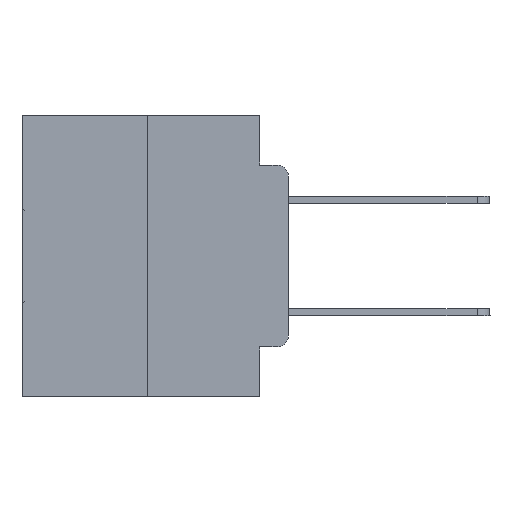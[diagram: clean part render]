
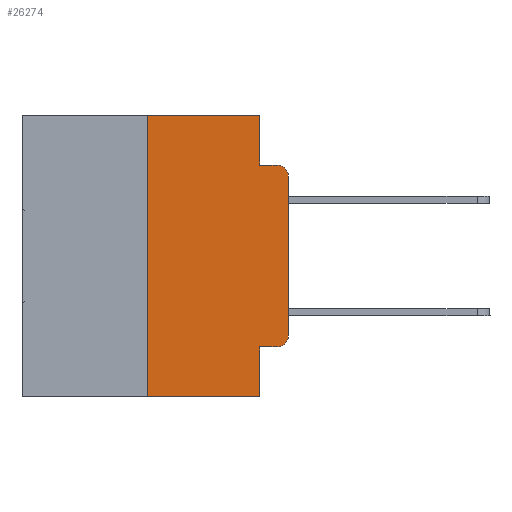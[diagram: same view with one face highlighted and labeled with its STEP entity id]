
A CAD part, left-side view. The second image highlights one B-rep face of the part: STEP entity #26274.
In plain terms, the highlighted planar face has unit normal (-1, 0, 0).
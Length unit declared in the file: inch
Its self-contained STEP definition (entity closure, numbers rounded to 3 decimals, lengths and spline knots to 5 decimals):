
#2 = CARTESIAN_POINT ( 'NONE',  ( 0., 0.051, -0.4115 ) ) ;
#1365 = CARTESIAN_POINT ( 'NONE',  ( 0., 0.051, 0. ) ) ;
#1436 = DIRECTION ( 'NONE',  ( -1., 0., 0. ) ) ;
#1447 = VECTOR ( 'NONE', #6251, 39.37008 ) ;
#1480 = DIRECTION ( 'NONE',  ( 0., 0., -1. ) ) ;
#2574 = DIRECTION ( 'NONE',  ( 0., -1., 0. ) ) ;
#2601 = LINE ( 'NONE', #25767, #10209 ) ;
#2672 = VECTOR ( 'NONE', #25219, 39.37008 ) ;
#3342 = CARTESIAN_POINT ( 'NONE',  ( 0., 0.473, -0.5 ) ) ;
#3492 = VERTEX_POINT ( 'NONE', #8586 ) ;
#4495 = ORIENTED_EDGE ( 'NONE', *, *, #32081, .T. ) ;
#4887 = LINE ( 'NONE', #1365, #26101 ) ;
#4944 = VECTOR ( 'NONE', #2574, 39.37008 ) ;
#5983 = EDGE_CURVE ( 'NONE', #24963, #23833, #2601, .T. ) ;
#6019 = CARTESIAN_POINT ( 'NONE',  ( 0., 0.051, -0.0885 ) ) ;
#6251 = DIRECTION ( 'NONE',  ( 0., -1., 0. ) ) ;
#7625 = CARTESIAN_POINT ( 'NONE',  ( 0., 0.051, -0.0885 ) ) ;
#8046 = VECTOR ( 'NONE', #30836, 39.37008 ) ;
#8366 = CARTESIAN_POINT ( 'NONE',  ( 0., 0.051, -0.4115 ) ) ;
#8586 = CARTESIAN_POINT ( 'NONE',  ( 0., 0., -0.3915 ) ) ;
#8615 = VERTEX_POINT ( 'NONE', #16525 ) ;
#8672 = CARTESIAN_POINT ( 'NONE',  ( 0., 0.473, 0. ) ) ;
#9557 = ORIENTED_EDGE ( 'NONE', *, *, #26837, .T. ) ;
#10017 = DIRECTION ( 'NONE',  ( -1., 0., 0. ) ) ;
#10176 = ORIENTED_EDGE ( 'NONE', *, *, #13258, .F. ) ;
#10209 = VECTOR ( 'NONE', #20400, 39.37008 ) ;
#10474 = AXIS2_PLACEMENT_3D ( 'NONE', #28047, #10017, #20224 ) ;
#12135 = AXIS2_PLACEMENT_3D ( 'NONE', #26826, #1436, #16648 ) ;
#12227 = VECTOR ( 'NONE', #26302, 39.37008 ) ;
#12442 = CARTESIAN_POINT ( 'NONE',  ( 0., 0.25, -0.5 ) ) ;
#12909 = CARTESIAN_POINT ( 'NONE',  ( 0., 0.02, -0.4115 ) ) ;
#13196 = EDGE_CURVE ( 'NONE', #17212, #8615, #16471, .T. ) ;
#13258 = EDGE_CURVE ( 'NONE', #15670, #23343, #27294, .T. ) ;
#14021 = ORIENTED_EDGE ( 'NONE', *, *, #20124, .T. ) ;
#15471 = LINE ( 'NONE', #8366, #1447 ) ;
#15670 = VERTEX_POINT ( 'NONE', #2 ) ;
#16412 = DIRECTION ( 'NONE',  ( 0., 0., -1. ) ) ;
#16471 = CIRCLE ( 'NONE', #10474, 0.02 ) ;
#16525 = CARTESIAN_POINT ( 'NONE',  ( 0., 0.02, -0.0885 ) ) ;
#16648 = DIRECTION ( 'NONE',  ( 0., 0., -1. ) ) ;
#17212 = VERTEX_POINT ( 'NONE', #27606 ) ;
#18235 = LINE ( 'NONE', #18359, #28618 ) ;
#18359 = CARTESIAN_POINT ( 'NONE',  ( 0., 0., 0. ) ) ;
#19729 = ORIENTED_EDGE ( 'NONE', *, *, #13196, .T. ) ;
#19916 = CARTESIAN_POINT ( 'NONE',  ( 0., 0.051, 0. ) ) ;
#20124 = EDGE_CURVE ( 'NONE', #28458, #23343, #22621, .T. ) ;
#20161 = VERTEX_POINT ( 'NONE', #6019 ) ;
#20224 = DIRECTION ( 'NONE',  ( 0., 0., -1. ) ) ;
#20400 = DIRECTION ( 'NONE',  ( 0., -1., 0. ) ) ;
#20582 = ORIENTED_EDGE ( 'NONE', *, *, #5983, .F. ) ;
#20632 = VERTEX_POINT ( 'NONE', #12909 ) ;
#21016 = ORIENTED_EDGE ( 'NONE', *, *, #22780, .F. ) ;
#21095 = EDGE_CURVE ( 'NONE', #20161, #8615, #23353, .T. ) ;
#22062 = ORIENTED_EDGE ( 'NONE', *, *, #23062, .T. ) ;
#22621 = LINE ( 'NONE', #3342, #12227 ) ;
#22780 = EDGE_CURVE ( 'NONE', #23833, #20161, #4887, .T. ) ;
#23062 = EDGE_CURVE ( 'NONE', #15670, #20632, #15471, .T. ) ;
#23343 = VERTEX_POINT ( 'NONE', #30082 ) ;
#23353 = LINE ( 'NONE', #7625, #4944 ) ;
#23796 = ORIENTED_EDGE ( 'NONE', *, *, #30231, .F. ) ;
#23833 = VERTEX_POINT ( 'NONE', #19916 ) ;
#23997 = PLANE ( 'NONE',  #29926 ) ;
#24219 = DIRECTION ( 'NONE',  ( 1., 0., 0. ) ) ;
#24963 = VERTEX_POINT ( 'NONE', #29328 ) ;
#25219 = DIRECTION ( 'NONE',  ( 0., 0., 1. ) ) ;
#25767 = CARTESIAN_POINT ( 'NONE',  ( 0., 0.473, 0. ) ) ;
#26074 = DIRECTION ( 'NONE',  ( 0., 0., 1. ) ) ;
#26101 = VECTOR ( 'NONE', #1480, 39.37008 ) ;
#26274 = ADVANCED_FACE ( 'NONE', ( #27096 ), #23997, .F. ) ;
#26302 = DIRECTION ( 'NONE',  ( 0., -1., 0. ) ) ;
#26826 = CARTESIAN_POINT ( 'NONE',  ( 0., 0.02, -0.3915 ) ) ;
#26837 = EDGE_CURVE ( 'NONE', #20632, #3492, #29080, .T. ) ;
#27096 = FACE_OUTER_BOUND ( 'NONE', #29685, .T. ) ;
#27294 = LINE ( 'NONE', #32991, #8046 ) ;
#27606 = CARTESIAN_POINT ( 'NONE',  ( 0., 0., -0.1085 ) ) ;
#28047 = CARTESIAN_POINT ( 'NONE',  ( 0., 0.02, -0.1085 ) ) ;
#28114 = ORIENTED_EDGE ( 'NONE', *, *, #21095, .F. ) ;
#28458 = VERTEX_POINT ( 'NONE', #12442 ) ;
#28618 = VECTOR ( 'NONE', #26074, 39.37008 ) ;
#29080 = CIRCLE ( 'NONE', #12135, 0.02 ) ;
#29328 = CARTESIAN_POINT ( 'NONE',  ( 0., 0.25, 0. ) ) ;
#29685 = EDGE_LOOP ( 'NONE', ( #4495, #19729, #28114, #21016, #20582, #23796, #14021, #10176, #22062, #9557 ) ) ;
#29926 = AXIS2_PLACEMENT_3D ( 'NONE', #8672, #24219, #16412 ) ;
#30082 = CARTESIAN_POINT ( 'NONE',  ( 0., 0.051, -0.5 ) ) ;
#30123 = CARTESIAN_POINT ( 'NONE',  ( 0., 0.25, 0. ) ) ;
#30231 = EDGE_CURVE ( 'NONE', #28458, #24963, #30728, .T. ) ;
#30728 = LINE ( 'NONE', #30123, #2672 ) ;
#30836 = DIRECTION ( 'NONE',  ( 0., 0., -1. ) ) ;
#32081 = EDGE_CURVE ( 'NONE', #3492, #17212, #18235, .T. ) ;
#32991 = CARTESIAN_POINT ( 'NONE',  ( 0., 0.051, 0. ) ) ;
